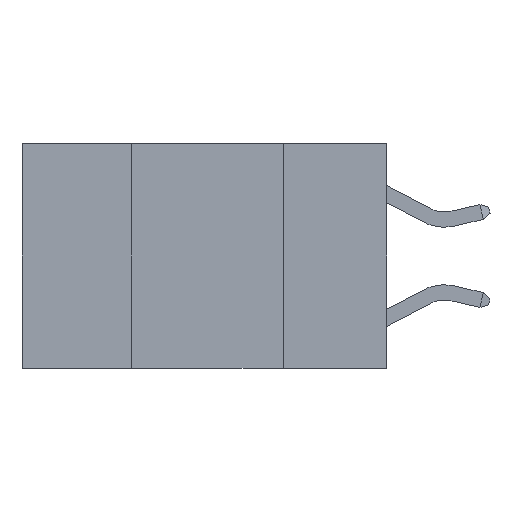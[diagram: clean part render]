
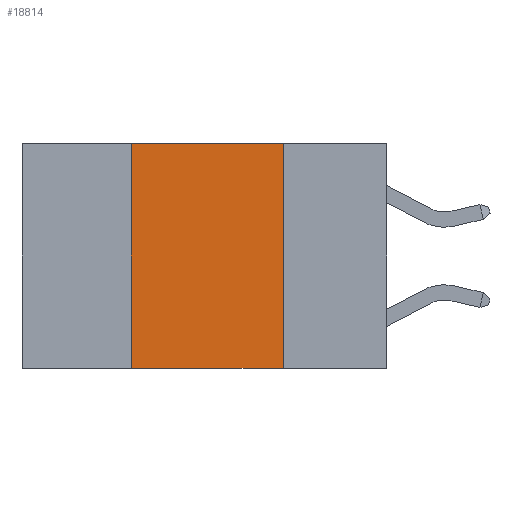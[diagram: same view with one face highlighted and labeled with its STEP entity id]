
A CAD part, left-side view. The second image highlights one B-rep face of the part: STEP entity #18814.
In plain terms, the highlighted planar face has unit normal (-1, 0, 0).
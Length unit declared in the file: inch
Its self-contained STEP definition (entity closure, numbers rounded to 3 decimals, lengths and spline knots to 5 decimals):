
#1864 = CARTESIAN_POINT ( 'NONE',  ( 0., 0.17, 0. ) ) ;
#1998 = ORIENTED_EDGE ( 'NONE', *, *, #20841, .F. ) ;
#2644 = EDGE_LOOP ( 'NONE', ( #13115, #1998, #12779, #18783 ) ) ;
#2949 = VECTOR ( 'NONE', #18247, 39.37008 ) ;
#3705 = PLANE ( 'NONE',  #16193 ) ;
#4383 = CARTESIAN_POINT ( 'NONE',  ( 0., 0.6, -0.37 ) ) ;
#4676 = LINE ( 'NONE', #11380, #12004 ) ;
#5472 = LINE ( 'NONE', #14144, #2949 ) ;
#5624 = CARTESIAN_POINT ( 'NONE',  ( 0., 0.17, -0.37 ) ) ;
#5927 = CARTESIAN_POINT ( 'NONE',  ( 0., 0.17, 0. ) ) ;
#6708 = VERTEX_POINT ( 'NONE', #5927 ) ;
#9867 = EDGE_CURVE ( 'NONE', #20409, #17839, #5472, .T. ) ;
#10523 = CARTESIAN_POINT ( 'NONE',  ( 0., 0.6, 0. ) ) ;
#11311 = DIRECTION ( 'NONE',  ( 0., -1., 0. ) ) ;
#11380 = CARTESIAN_POINT ( 'NONE',  ( 0., 0.6, 0. ) ) ;
#12004 = VECTOR ( 'NONE', #18142, 39.37008 ) ;
#12779 = ORIENTED_EDGE ( 'NONE', *, *, #9867, .F. ) ;
#13115 = ORIENTED_EDGE ( 'NONE', *, *, #16359, .F. ) ;
#14000 = DIRECTION ( 'NONE',  ( 0., 0., -1. ) ) ;
#14144 = CARTESIAN_POINT ( 'NONE',  ( 0., 0.42, 0. ) ) ;
#14481 = VECTOR ( 'NONE', #11311, 39.37008 ) ;
#14611 = CARTESIAN_POINT ( 'NONE',  ( 0., 0.42, -0.37 ) ) ;
#15671 = LINE ( 'NONE', #1864, #17575 ) ;
#15841 = DIRECTION ( 'NONE',  ( 1., 0., 0. ) ) ;
#16193 = AXIS2_PLACEMENT_3D ( 'NONE', #10523, #15841, #20854 ) ;
#16359 = EDGE_CURVE ( 'NONE', #6708, #21430, #15671, .T. ) ;
#17575 = VECTOR ( 'NONE', #14000, 39.37008 ) ;
#17839 = VERTEX_POINT ( 'NONE', #21017 ) ;
#18142 = DIRECTION ( 'NONE',  ( 0., -1., 0. ) ) ;
#18247 = DIRECTION ( 'NONE',  ( 0., 0., 1. ) ) ;
#18783 = ORIENTED_EDGE ( 'NONE', *, *, #21554, .T. ) ;
#18814 = ADVANCED_FACE ( 'NONE', ( #19385 ), #3705, .F. ) ;
#19385 = FACE_OUTER_BOUND ( 'NONE', #2644, .T. ) ;
#19635 = LINE ( 'NONE', #4383, #14481 ) ;
#20409 = VERTEX_POINT ( 'NONE', #14611 ) ;
#20841 = EDGE_CURVE ( 'NONE', #17839, #6708, #4676, .T. ) ;
#20854 = DIRECTION ( 'NONE',  ( 0., 0., -1. ) ) ;
#21017 = CARTESIAN_POINT ( 'NONE',  ( 0., 0.42, 0. ) ) ;
#21430 = VERTEX_POINT ( 'NONE', #5624 ) ;
#21554 = EDGE_CURVE ( 'NONE', #20409, #21430, #19635, .T. ) ;
